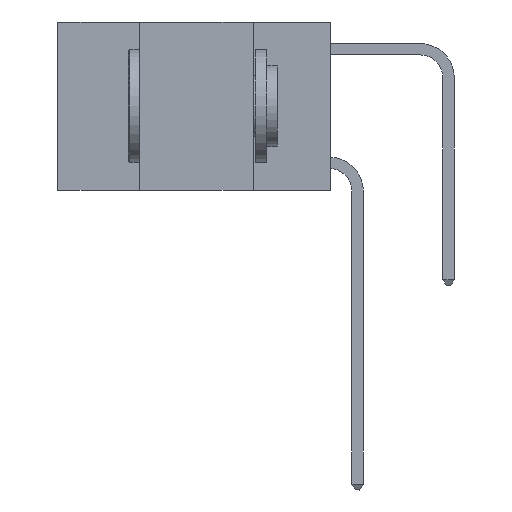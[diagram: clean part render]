
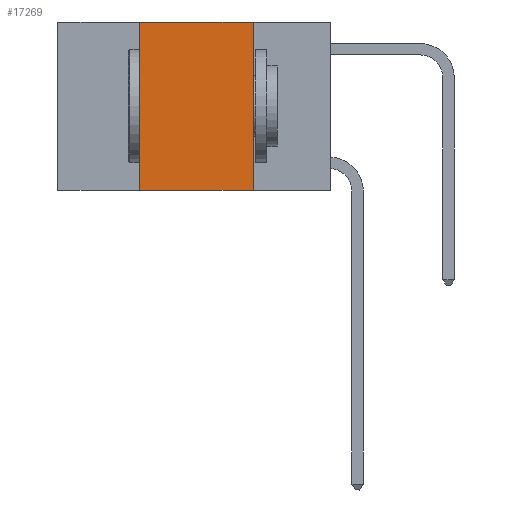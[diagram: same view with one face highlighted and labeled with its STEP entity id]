
A CAD part, left-side view. The second image highlights one B-rep face of the part: STEP entity #17269.
In plain terms, the highlighted planar face has unit normal (-1, 0, 0).
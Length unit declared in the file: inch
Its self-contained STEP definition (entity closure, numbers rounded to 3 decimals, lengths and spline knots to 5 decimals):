
#1042 = DIRECTION ( 'NONE',  ( 0., 0., -1. ) ) ;
#1074 = ORIENTED_EDGE ( 'NONE', *, *, #21769, .F. ) ;
#1205 = DIRECTION ( 'NONE',  ( 1., 0., 0. ) ) ;
#1511 = VERTEX_POINT ( 'NONE', #6227 ) ;
#1562 = DIRECTION ( 'NONE',  ( 0., 0., -1. ) ) ;
#1766 = DIRECTION ( 'NONE',  ( 0., -1., 0. ) ) ;
#2765 = CARTESIAN_POINT ( 'NONE',  ( 0., 0.42, -0.37 ) ) ;
#5907 = FACE_OUTER_BOUND ( 'NONE', #27953, .T. ) ;
#6227 = CARTESIAN_POINT ( 'NONE',  ( 0., 0.17, 0. ) ) ;
#7160 = VECTOR ( 'NONE', #27522, 39.37008 ) ;
#10190 = CARTESIAN_POINT ( 'NONE',  ( 0., 0.42, 0. ) ) ;
#10847 = VECTOR ( 'NONE', #1766, 39.37008 ) ;
#10986 = EDGE_CURVE ( 'NONE', #16584, #1511, #19105, .T. ) ;
#11100 = VECTOR ( 'NONE', #1562, 39.37008 ) ;
#12784 = LINE ( 'NONE', #10190, #7160 ) ;
#13832 = CARTESIAN_POINT ( 'NONE',  ( 0., 0.6, 0. ) ) ;
#16150 = CARTESIAN_POINT ( 'NONE',  ( 0., 0.6, -0.37 ) ) ;
#16584 = VERTEX_POINT ( 'NONE', #19759 ) ;
#17269 = ADVANCED_FACE ( 'NONE', ( #5907 ), #30541, .F. ) ;
#18504 = EDGE_CURVE ( 'NONE', #1511, #31195, #30912, .T. ) ;
#19105 = LINE ( 'NONE', #26391, #10847 ) ;
#19676 = VERTEX_POINT ( 'NONE', #2765 ) ;
#19759 = CARTESIAN_POINT ( 'NONE',  ( 0., 0.42, 0. ) ) ;
#21769 = EDGE_CURVE ( 'NONE', #19676, #16584, #12784, .T. ) ;
#22055 = DIRECTION ( 'NONE',  ( 0., -1., 0. ) ) ;
#22949 = AXIS2_PLACEMENT_3D ( 'NONE', #13832, #1205, #1042 ) ;
#23123 = CARTESIAN_POINT ( 'NONE',  ( 0., 0.17, 0. ) ) ;
#24316 = ORIENTED_EDGE ( 'NONE', *, *, #18504, .F. ) ;
#24418 = CARTESIAN_POINT ( 'NONE',  ( 0., 0.17, -0.37 ) ) ;
#25607 = ORIENTED_EDGE ( 'NONE', *, *, #10986, .F. ) ;
#26145 = VECTOR ( 'NONE', #22055, 39.37008 ) ;
#26391 = CARTESIAN_POINT ( 'NONE',  ( 0., 0.6, 0. ) ) ;
#27522 = DIRECTION ( 'NONE',  ( 0., 0., 1. ) ) ;
#27953 = EDGE_LOOP ( 'NONE', ( #24316, #25607, #1074, #29094 ) ) ;
#29094 = ORIENTED_EDGE ( 'NONE', *, *, #31399, .T. ) ;
#30541 = PLANE ( 'NONE',  #22949 ) ;
#30581 = LINE ( 'NONE', #16150, #26145 ) ;
#30912 = LINE ( 'NONE', #23123, #11100 ) ;
#31195 = VERTEX_POINT ( 'NONE', #24418 ) ;
#31399 = EDGE_CURVE ( 'NONE', #19676, #31195, #30581, .T. ) ;
